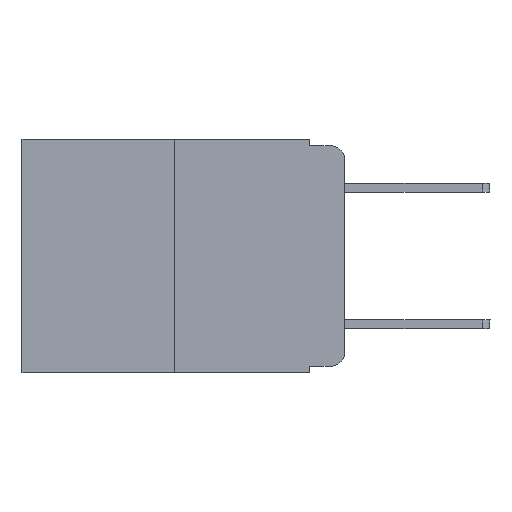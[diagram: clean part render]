
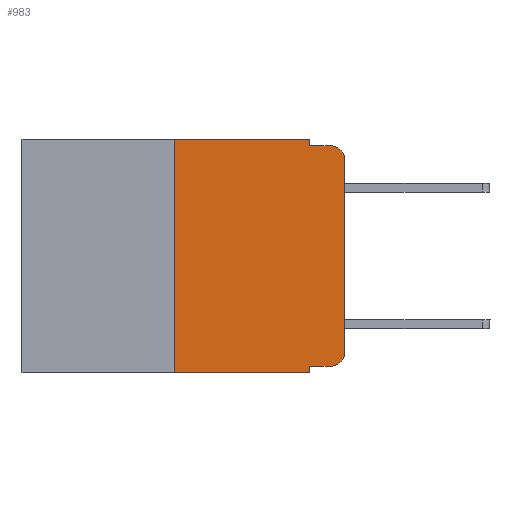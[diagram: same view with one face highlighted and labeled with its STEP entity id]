
A CAD part, left-side view. The second image highlights one B-rep face of the part: STEP entity #983.
In plain terms, the highlighted planar face has unit normal (-1, 0, 0).
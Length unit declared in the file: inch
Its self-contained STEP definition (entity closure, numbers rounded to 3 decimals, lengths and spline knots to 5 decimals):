
#134 = CARTESIAN_POINT ( 'NONE',  ( 0., 0.02, -0.313 ) ) ;
#891 = VERTEX_POINT ( 'NONE', #3677 ) ;
#983 = ADVANCED_FACE ( 'NONE', ( #12249 ), #17896, .F. ) ;
#1179 = CARTESIAN_POINT ( 'NONE',  ( 0., 0.051, -0.343 ) ) ;
#1214 = DIRECTION ( 'NONE',  ( 0., 0., -1. ) ) ;
#1305 = DIRECTION ( 'NONE',  ( 0., 0., 1. ) ) ;
#1469 = LINE ( 'NONE', #2706, #7501 ) ;
#1596 = EDGE_CURVE ( 'NONE', #14431, #10318, #14923, .T. ) ;
#1643 = ORIENTED_EDGE ( 'NONE', *, *, #17188, .F. ) ;
#1899 = CARTESIAN_POINT ( 'NONE',  ( 0., 0.473, 0. ) ) ;
#1951 = VERTEX_POINT ( 'NONE', #15129 ) ;
#2318 = CARTESIAN_POINT ( 'NONE',  ( 0., 0.02, -0.03 ) ) ;
#2406 = CARTESIAN_POINT ( 'NONE',  ( 0., 0., -0.313 ) ) ;
#2519 = EDGE_LOOP ( 'NONE', ( #12664, #14407, #7330, #17607, #1643, #4288, #8831, #17446, #6179, #8721 ) ) ;
#2701 = VECTOR ( 'NONE', #17460, 39.37008 ) ;
#2706 = CARTESIAN_POINT ( 'NONE',  ( 0., 0., 0. ) ) ;
#3118 = EDGE_CURVE ( 'NONE', #891, #11617, #15513, .T. ) ;
#3677 = CARTESIAN_POINT ( 'NONE',  ( 0., 0.051, 0. ) ) ;
#3702 = EDGE_CURVE ( 'NONE', #11617, #1951, #16500, .T. ) ;
#3980 = CARTESIAN_POINT ( 'NONE',  ( 0., 0.051, 0. ) ) ;
#4037 = EDGE_CURVE ( 'NONE', #10225, #9746, #1469, .T. ) ;
#4183 = DIRECTION ( 'NONE',  ( -1., 0., 0. ) ) ;
#4288 = ORIENTED_EDGE ( 'NONE', *, *, #11196, .F. ) ;
#4510 = CARTESIAN_POINT ( 'NONE',  ( 0., 0.051, -0.333 ) ) ;
#5263 = VERTEX_POINT ( 'NONE', #4510 ) ;
#5813 = VECTOR ( 'NONE', #1214, 39.37008 ) ;
#6147 = VECTOR ( 'NONE', #9106, 39.37008 ) ;
#6179 = ORIENTED_EDGE ( 'NONE', *, *, #11266, .T. ) ;
#7187 = CARTESIAN_POINT ( 'NONE',  ( 0., 0.473, 0. ) ) ;
#7233 = AXIS2_PLACEMENT_3D ( 'NONE', #1899, #9342, #15070 ) ;
#7330 = ORIENTED_EDGE ( 'NONE', *, *, #3702, .F. ) ;
#7410 = CARTESIAN_POINT ( 'NONE',  ( 0., 0.473, -0.343 ) ) ;
#7501 = VECTOR ( 'NONE', #14178, 39.37008 ) ;
#8003 = CARTESIAN_POINT ( 'NONE',  ( 0., 0., -0.03 ) ) ;
#8376 = CARTESIAN_POINT ( 'NONE',  ( 0., 0.051, 0. ) ) ;
#8721 = ORIENTED_EDGE ( 'NONE', *, *, #16265, .T. ) ;
#8831 = ORIENTED_EDGE ( 'NONE', *, *, #1596, .T. ) ;
#9039 = VECTOR ( 'NONE', #1305, 39.37008 ) ;
#9106 = DIRECTION ( 'NONE',  ( 0., -1., 0. ) ) ;
#9342 = DIRECTION ( 'NONE',  ( 1., 0., 0. ) ) ;
#9437 = CARTESIAN_POINT ( 'NONE',  ( 0., 0.051, -0.01 ) ) ;
#9519 = VECTOR ( 'NONE', #14151, 39.37008 ) ;
#9746 = VERTEX_POINT ( 'NONE', #8003 ) ;
#9969 = DIRECTION ( 'NONE',  ( 0., 0., -1. ) ) ;
#10144 = CIRCLE ( 'NONE', #18550, 0.02 ) ;
#10225 = VERTEX_POINT ( 'NONE', #2406 ) ;
#10318 = VERTEX_POINT ( 'NONE', #1179 ) ;
#11074 = VECTOR ( 'NONE', #18000, 39.37008 ) ;
#11196 = EDGE_CURVE ( 'NONE', #14431, #15430, #11495, .T. ) ;
#11266 = EDGE_CURVE ( 'NONE', #5263, #12966, #15895, .T. ) ;
#11495 = LINE ( 'NONE', #15790, #9039 ) ;
#11617 = VERTEX_POINT ( 'NONE', #17945 ) ;
#11753 = AXIS2_PLACEMENT_3D ( 'NONE', #134, #4183, #9969 ) ;
#12193 = EDGE_CURVE ( 'NONE', #5263, #10318, #18306, .T. ) ;
#12249 = FACE_OUTER_BOUND ( 'NONE', #2519, .T. ) ;
#12372 = VECTOR ( 'NONE', #18437, 39.37008 ) ;
#12639 = CIRCLE ( 'NONE', #11753, 0.02 ) ;
#12664 = ORIENTED_EDGE ( 'NONE', *, *, #4037, .T. ) ;
#12699 = CARTESIAN_POINT ( 'NONE',  ( 0., 0.051, -0.333 ) ) ;
#12966 = VERTEX_POINT ( 'NONE', #14849 ) ;
#13077 = EDGE_CURVE ( 'NONE', #9746, #1951, #10144, .T. ) ;
#14151 = DIRECTION ( 'NONE',  ( 0., 0., -1. ) ) ;
#14178 = DIRECTION ( 'NONE',  ( 0., 0., 1. ) ) ;
#14407 = ORIENTED_EDGE ( 'NONE', *, *, #13077, .T. ) ;
#14431 = VERTEX_POINT ( 'NONE', #15130 ) ;
#14495 = CARTESIAN_POINT ( 'NONE',  ( 0., 0.25, 0. ) ) ;
#14849 = CARTESIAN_POINT ( 'NONE',  ( 0., 0.02, -0.333 ) ) ;
#14923 = LINE ( 'NONE', #7410, #6147 ) ;
#15049 = DIRECTION ( 'NONE',  ( -1., 0., 0. ) ) ;
#15070 = DIRECTION ( 'NONE',  ( 0., 0., -1. ) ) ;
#15129 = CARTESIAN_POINT ( 'NONE',  ( 0., 0.02, -0.01 ) ) ;
#15130 = CARTESIAN_POINT ( 'NONE',  ( 0., 0.25, -0.343 ) ) ;
#15430 = VERTEX_POINT ( 'NONE', #14495 ) ;
#15513 = LINE ( 'NONE', #8376, #5813 ) ;
#15790 = CARTESIAN_POINT ( 'NONE',  ( 0., 0.25, 0. ) ) ;
#15895 = LINE ( 'NONE', #12699, #12372 ) ;
#16265 = EDGE_CURVE ( 'NONE', #12966, #10225, #12639, .T. ) ;
#16500 = LINE ( 'NONE', #9437, #11074 ) ;
#16566 = DIRECTION ( 'NONE',  ( 0., 0., -1. ) ) ;
#17081 = LINE ( 'NONE', #7187, #2701 ) ;
#17188 = EDGE_CURVE ( 'NONE', #15430, #891, #17081, .T. ) ;
#17446 = ORIENTED_EDGE ( 'NONE', *, *, #12193, .F. ) ;
#17460 = DIRECTION ( 'NONE',  ( 0., -1., 0. ) ) ;
#17607 = ORIENTED_EDGE ( 'NONE', *, *, #3118, .F. ) ;
#17896 = PLANE ( 'NONE',  #7233 ) ;
#17945 = CARTESIAN_POINT ( 'NONE',  ( 0., 0.051, -0.01 ) ) ;
#18000 = DIRECTION ( 'NONE',  ( 0., -1., 0. ) ) ;
#18306 = LINE ( 'NONE', #3980, #9519 ) ;
#18437 = DIRECTION ( 'NONE',  ( 0., -1., 0. ) ) ;
#18550 = AXIS2_PLACEMENT_3D ( 'NONE', #2318, #15049, #16566 ) ;
